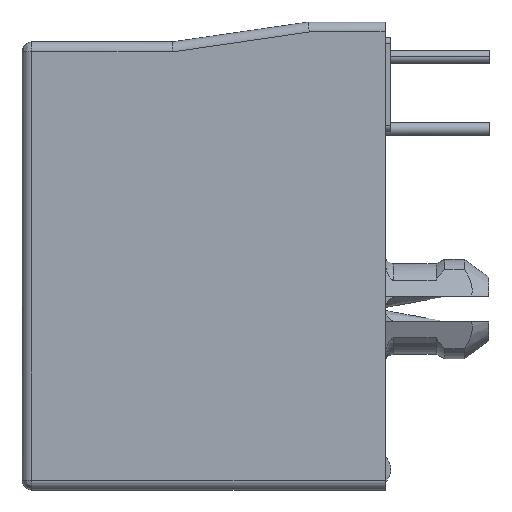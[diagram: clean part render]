
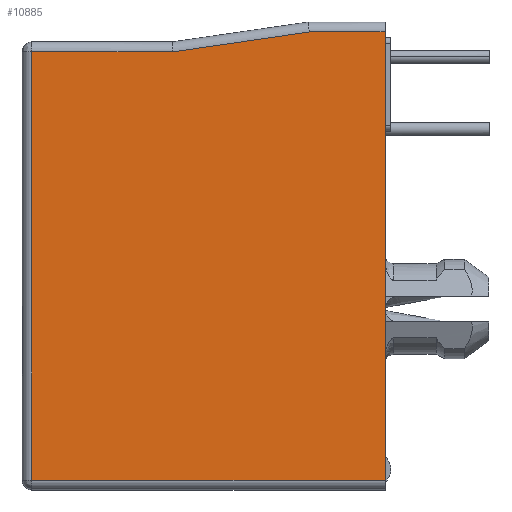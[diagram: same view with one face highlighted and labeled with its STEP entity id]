
A CAD part, left-side view. The second image highlights one B-rep face of the part: STEP entity #10885.
In plain terms, the highlighted planar face has unit normal (-1, 0, 0).
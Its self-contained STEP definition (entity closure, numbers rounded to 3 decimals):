
#568 = DIRECTION ( 'NONE',  ( 0., 1., 0. ) ) ;
#2263 = ORIENTED_EDGE ( 'NONE', *, *, #5698, .T. ) ;
#2460 = VERTEX_POINT ( 'NONE', #19788 ) ;
#3450 = DIRECTION ( 'NONE',  ( 0., -1., 0. ) ) ;
#4068 = EDGE_CURVE ( 'NONE', #5560, #2460, #5615, .T. ) ;
#4544 = CARTESIAN_POINT ( 'NONE',  ( -7.65, -4.825, 9.77 ) ) ;
#5065 = DIRECTION ( 'NONE',  ( 0., 0., 1. ) ) ;
#5207 = LINE ( 'NONE', #19008, #7557 ) ;
#5560 = VERTEX_POINT ( 'NONE', #19624 ) ;
#5615 = LINE ( 'NONE', #10354, #18076 ) ;
#5686 = LINE ( 'NONE', #18455, #17094 ) ;
#5698 = EDGE_CURVE ( 'NONE', #5560, #21392, #5746, .T. ) ;
#5746 = LINE ( 'NONE', #11874, #15596 ) ;
#6439 = DIRECTION ( 'NONE',  ( 0., -0.99, 0.144 ) ) ;
#7107 = PLANE ( 'NONE',  #18947 ) ;
#7557 = VECTOR ( 'NONE', #12451, 1000. ) ;
#7938 = EDGE_LOOP ( 'NONE', ( #21436, #2263, #8535, #16058, #15358, #9987 ) ) ;
#8162 = CARTESIAN_POINT ( 'NONE',  ( -7.65, 7.625, 1.87 ) ) ;
#8474 = CARTESIAN_POINT ( 'NONE',  ( -7.65, -2.15, 9.77 ) ) ;
#8535 = ORIENTED_EDGE ( 'NONE', *, *, #17687, .F. ) ;
#9180 = CARTESIAN_POINT ( 'NONE',  ( -7.65, 7.625, 9.07 ) ) ;
#9987 = ORIENTED_EDGE ( 'NONE', *, *, #18616, .F. ) ;
#10354 = CARTESIAN_POINT ( 'NONE',  ( -7.65, 1.4, -6.03 ) ) ;
#10885 = ADVANCED_FACE ( 'NONE', ( #20090 ), #7107, .T. ) ;
#11036 = VERTEX_POINT ( 'NONE', #9180 ) ;
#11496 = VECTOR ( 'NONE', #6439, 1000. ) ;
#11512 = CARTESIAN_POINT ( 'NONE',  ( -7.65, 2.65, 9.07 ) ) ;
#11874 = CARTESIAN_POINT ( 'NONE',  ( -7.65, -4.825, 10.086 ) ) ;
#12451 = DIRECTION ( 'NONE',  ( 0., -1., 0. ) ) ;
#15204 = DIRECTION ( 'NONE',  ( 0., 1., 0. ) ) ;
#15358 = ORIENTED_EDGE ( 'NONE', *, *, #17089, .F. ) ;
#15596 = VECTOR ( 'NONE', #5065, 1000. ) ;
#16058 = ORIENTED_EDGE ( 'NONE', *, *, #21349, .F. ) ;
#16860 = VERTEX_POINT ( 'NONE', #8474 ) ;
#16910 = VERTEX_POINT ( 'NONE', #11512 ) ;
#17089 = EDGE_CURVE ( 'NONE', #11036, #16910, #5207, .T. ) ;
#17094 = VECTOR ( 'NONE', #3450, 1000. ) ;
#17687 = EDGE_CURVE ( 'NONE', #16860, #21392, #5686, .T. ) ;
#17797 = CARTESIAN_POINT ( 'NONE',  ( -7.65, -2.204, 9.778 ) ) ;
#18076 = VECTOR ( 'NONE', #15204, 1000. ) ;
#18455 = CARTESIAN_POINT ( 'NONE',  ( -7.65, 1.4, 9.77 ) ) ;
#18524 = DIRECTION ( 'NONE',  ( -1., 0., 0. ) ) ;
#18616 = EDGE_CURVE ( 'NONE', #2460, #11036, #21440, .T. ) ;
#18947 = AXIS2_PLACEMENT_3D ( 'NONE', #20260, #18524, #568 ) ;
#19008 = CARTESIAN_POINT ( 'NONE',  ( -7.65, 1.4, 9.07 ) ) ;
#19123 = VECTOR ( 'NONE', #19513, 1000. ) ;
#19513 = DIRECTION ( 'NONE',  ( 0., 0., 1. ) ) ;
#19624 = CARTESIAN_POINT ( 'NONE',  ( -7.65, -4.825, -6.03 ) ) ;
#19788 = CARTESIAN_POINT ( 'NONE',  ( -7.65, 7.625, -6.03 ) ) ;
#20090 = FACE_OUTER_BOUND ( 'NONE', #7938, .T. ) ;
#20260 = CARTESIAN_POINT ( 'NONE',  ( -7.65, -5.074, 10.086 ) ) ;
#21073 = LINE ( 'NONE', #17797, #11496 ) ;
#21349 = EDGE_CURVE ( 'NONE', #16910, #16860, #21073, .T. ) ;
#21392 = VERTEX_POINT ( 'NONE', #4544 ) ;
#21436 = ORIENTED_EDGE ( 'NONE', *, *, #4068, .F. ) ;
#21440 = LINE ( 'NONE', #8162, #19123 ) ;
